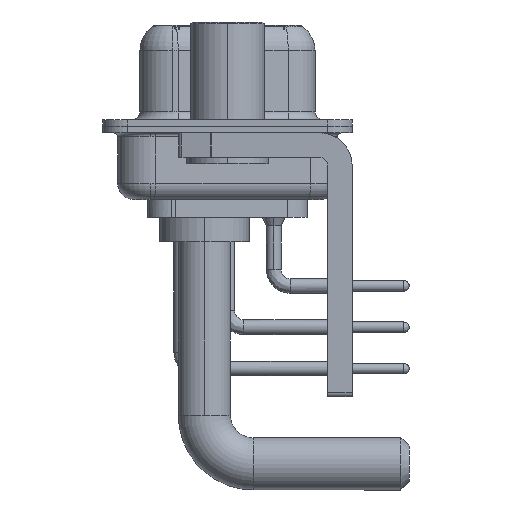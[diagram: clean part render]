
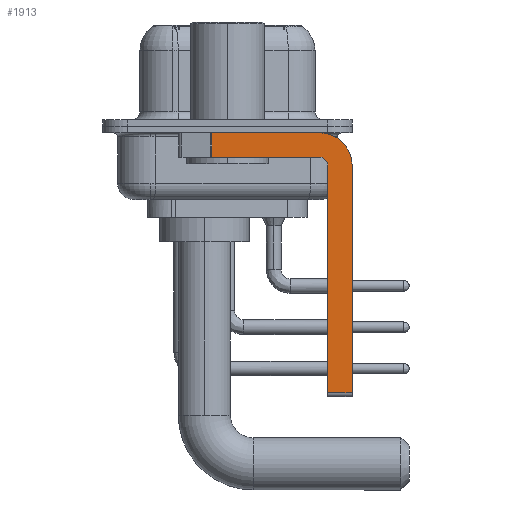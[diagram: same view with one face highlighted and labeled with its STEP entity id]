
A CAD part, left-side view. The second image highlights one B-rep face of the part: STEP entity #1913.
In plain terms, the highlighted planar face has unit normal (-1, 0, 0).
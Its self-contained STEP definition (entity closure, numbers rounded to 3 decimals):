
#87 = CARTESIAN_POINT ( 'NONE',  ( -2.9, -7.65, -2.4 ) ) ;
#1913 = ADVANCED_FACE ( 'NONE', ( #3316 ), #25216, .F. ) ;
#2352 = LINE ( 'NONE', #87, #14316 ) ;
#3316 = FACE_OUTER_BOUND ( 'NONE', #30143, .T. ) ;
#3701 = VERTEX_POINT ( 'NONE', #24242 ) ;
#4264 = LINE ( 'NONE', #9123, #27001 ) ;
#5043 = EDGE_CURVE ( 'NONE', #30023, #20752, #2352, .T. ) ;
#5795 = LINE ( 'NONE', #20785, #18889 ) ;
#5848 = CIRCLE ( 'NONE', #30050, 0.5 ) ;
#5884 = DIRECTION ( 'NONE',  ( 0., 0., -1. ) ) ;
#7900 = DIRECTION ( 'NONE',  ( 0., 0., -1. ) ) ;
#8004 = ORIENTED_EDGE ( 'NONE', *, *, #22407, .T. ) ;
#8404 = CARTESIAN_POINT ( 'NONE',  ( -2.9, -5.65, -1.9 ) ) ;
#8497 = DIRECTION ( 'NONE',  ( 0., 0., 1. ) ) ;
#9123 = CARTESIAN_POINT ( 'NONE',  ( -2.9, -6.15, -16.6 ) ) ;
#9190 = LINE ( 'NONE', #21584, #10830 ) ;
#9488 = VERTEX_POINT ( 'NONE', #27074 ) ;
#10481 = DIRECTION ( 'NONE',  ( 1., 0., 0. ) ) ;
#10830 = VECTOR ( 'NONE', #13999, 1000. ) ;
#10855 = CARTESIAN_POINT ( 'NONE',  ( -2.9, 0.978, -0.4 ) ) ;
#10917 = ORIENTED_EDGE ( 'NONE', *, *, #14296, .F. ) ;
#11193 = LINE ( 'NONE', #13144, #12050 ) ;
#11555 = EDGE_CURVE ( 'NONE', #3701, #9488, #4264, .T. ) ;
#11603 = ORIENTED_EDGE ( 'NONE', *, *, #27224, .F. ) ;
#12050 = VECTOR ( 'NONE', #21009, 1000. ) ;
#12252 = CARTESIAN_POINT ( 'NONE',  ( -2.9, -5.65, -2.4 ) ) ;
#12264 = CARTESIAN_POINT ( 'NONE',  ( -2.9, -7.65, -16.35 ) ) ;
#13042 = VERTEX_POINT ( 'NONE', #19943 ) ;
#13144 = CARTESIAN_POINT ( 'NONE',  ( -2.9, 3., -0.4 ) ) ;
#13293 = EDGE_CURVE ( 'NONE', #3701, #20752, #24082, .T. ) ;
#13900 = ORIENTED_EDGE ( 'NONE', *, *, #5043, .F. ) ;
#13999 = DIRECTION ( 'NONE',  ( 0., 0., -1. ) ) ;
#14296 = EDGE_CURVE ( 'NONE', #21529, #30023, #16781, .T. ) ;
#14316 = VECTOR ( 'NONE', #25059, 1000. ) ;
#14371 = DIRECTION ( 'NONE',  ( 0., 0., 1. ) ) ;
#14695 = ORIENTED_EDGE ( 'NONE', *, *, #11555, .F. ) ;
#15423 = EDGE_CURVE ( 'NONE', #15895, #13042, #5795, .T. ) ;
#15678 = ORIENTED_EDGE ( 'NONE', *, *, #25688, .F. ) ;
#15895 = VERTEX_POINT ( 'NONE', #8404 ) ;
#16075 = CARTESIAN_POINT ( 'NONE',  ( -2.9, -7.65, -2.4 ) ) ;
#16721 = AXIS2_PLACEMENT_3D ( 'NONE', #23125, #27951, #5884 ) ;
#16781 = CIRCLE ( 'NONE', #28626, 2. ) ;
#18889 = VECTOR ( 'NONE', #30623, 1000. ) ;
#19943 = CARTESIAN_POINT ( 'NONE',  ( -2.9, 0.978, -1.9 ) ) ;
#20752 = VERTEX_POINT ( 'NONE', #12264 ) ;
#20785 = CARTESIAN_POINT ( 'NONE',  ( -2.9, -5.65, -1.9 ) ) ;
#21009 = DIRECTION ( 'NONE',  ( 0., -1., 0. ) ) ;
#21529 = VERTEX_POINT ( 'NONE', #26507 ) ;
#21584 = CARTESIAN_POINT ( 'NONE',  ( -2.9, 0.978, -1.9 ) ) ;
#21858 = VECTOR ( 'NONE', #26356, 1000. ) ;
#21954 = VERTEX_POINT ( 'NONE', #10855 ) ;
#22407 = EDGE_CURVE ( 'NONE', #21954, #13042, #9190, .T. ) ;
#23125 = CARTESIAN_POINT ( 'NONE',  ( -2.9, -5.65, -2.4 ) ) ;
#23311 = ORIENTED_EDGE ( 'NONE', *, *, #13293, .T. ) ;
#24082 = LINE ( 'NONE', #28919, #21858 ) ;
#24151 = ORIENTED_EDGE ( 'NONE', *, *, #15423, .F. ) ;
#24242 = CARTESIAN_POINT ( 'NONE',  ( -2.9, -6.15, -16.35 ) ) ;
#24682 = DIRECTION ( 'NONE',  ( -1., 0., 0. ) ) ;
#25059 = DIRECTION ( 'NONE',  ( 0., 0., -1. ) ) ;
#25216 = PLANE ( 'NONE',  #16721 ) ;
#25688 = EDGE_CURVE ( 'NONE', #9488, #15895, #5848, .T. ) ;
#26356 = DIRECTION ( 'NONE',  ( 0., -1., 0. ) ) ;
#26471 = CARTESIAN_POINT ( 'NONE',  ( -2.9, -5.65, -2.4 ) ) ;
#26507 = CARTESIAN_POINT ( 'NONE',  ( -2.9, -5.65, -0.4 ) ) ;
#27001 = VECTOR ( 'NONE', #8497, 1000. ) ;
#27074 = CARTESIAN_POINT ( 'NONE',  ( -2.9, -6.15, -2.4 ) ) ;
#27224 = EDGE_CURVE ( 'NONE', #21954, #21529, #11193, .T. ) ;
#27951 = DIRECTION ( 'NONE',  ( 1., 0., 0. ) ) ;
#28626 = AXIS2_PLACEMENT_3D ( 'NONE', #12252, #10481, #7900 ) ;
#28919 = CARTESIAN_POINT ( 'NONE',  ( -2.9, -5.65, -16.35 ) ) ;
#30023 = VERTEX_POINT ( 'NONE', #16075 ) ;
#30050 = AXIS2_PLACEMENT_3D ( 'NONE', #26471, #24682, #14371 ) ;
#30143 = EDGE_LOOP ( 'NONE', ( #11603, #8004, #24151, #15678, #14695, #23311, #13900, #10917 ) ) ;
#30623 = DIRECTION ( 'NONE',  ( 0., 1., 0. ) ) ;
